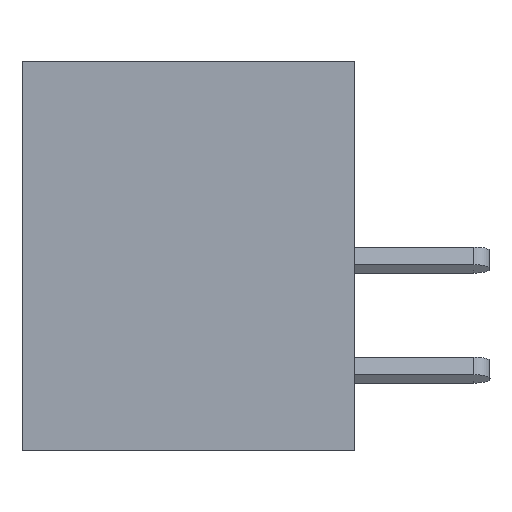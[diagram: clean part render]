
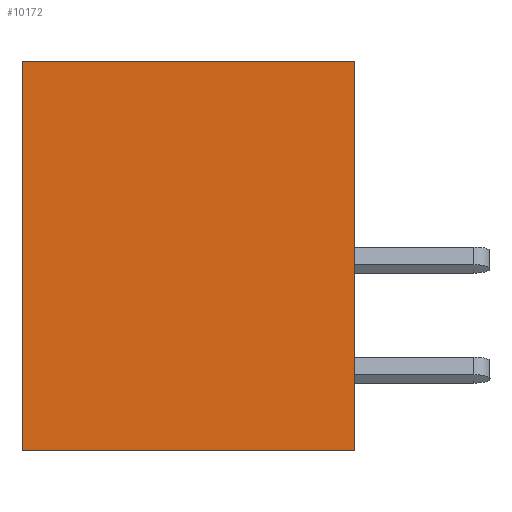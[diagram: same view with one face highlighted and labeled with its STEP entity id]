
A CAD part, left-side view. The second image highlights one B-rep face of the part: STEP entity #10172.
In plain terms, the highlighted planar face has unit normal (-1, 0, 0).
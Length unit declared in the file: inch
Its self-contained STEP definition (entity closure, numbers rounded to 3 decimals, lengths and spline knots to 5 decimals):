
#200 = CARTESIAN_POINT ( 'NONE',  ( 0., 0.453, 0. ) ) ;
#326 = LINE ( 'NONE', #12658, #6911 ) ;
#1226 = EDGE_CURVE ( 'NONE', #25572, #16957, #25368, .T. ) ;
#1540 = CARTESIAN_POINT ( 'NONE',  ( 0., 0.453, -0.531 ) ) ;
#1773 = CARTESIAN_POINT ( 'NONE',  ( 0., 0.453, 0. ) ) ;
#2562 = ORIENTED_EDGE ( 'NONE', *, *, #5221, .T. ) ;
#2761 = FACE_OUTER_BOUND ( 'NONE', #14135, .T. ) ;
#4261 = CARTESIAN_POINT ( 'NONE',  ( 0., 0.453, 0. ) ) ;
#5221 = EDGE_CURVE ( 'NONE', #15401, #17488, #27502, .T. ) ;
#6907 = DIRECTION ( 'NONE',  ( 0., -1., 0. ) ) ;
#6911 = VECTOR ( 'NONE', #14417, 39.37008 ) ;
#7282 = ORIENTED_EDGE ( 'NONE', *, *, #20754, .T. ) ;
#8296 = CARTESIAN_POINT ( 'NONE',  ( 0., 0., 0. ) ) ;
#10172 = ADVANCED_FACE ( 'NONE', ( #2761 ), #25554, .F. ) ;
#10483 = CARTESIAN_POINT ( 'NONE',  ( 0., 0.453, -0.531 ) ) ;
#11033 = ORIENTED_EDGE ( 'NONE', *, *, #1226, .F. ) ;
#12147 = VECTOR ( 'NONE', #6907, 39.37008 ) ;
#12658 = CARTESIAN_POINT ( 'NONE',  ( 0., 0., 0. ) ) ;
#12899 = DIRECTION ( 'NONE',  ( 0., 0., 1. ) ) ;
#14135 = EDGE_LOOP ( 'NONE', ( #7282, #11033, #19008, #2562 ) ) ;
#14417 = DIRECTION ( 'NONE',  ( 0., 0., 1. ) ) ;
#15272 = AXIS2_PLACEMENT_3D ( 'NONE', #20748, #21038, #18651 ) ;
#15401 = VERTEX_POINT ( 'NONE', #10483 ) ;
#15724 = VECTOR ( 'NONE', #18964, 39.37008 ) ;
#15932 = LINE ( 'NONE', #1773, #27024 ) ;
#16957 = VERTEX_POINT ( 'NONE', #8296 ) ;
#17488 = VERTEX_POINT ( 'NONE', #24282 ) ;
#18651 = DIRECTION ( 'NONE',  ( 0., 0., -1. ) ) ;
#18964 = DIRECTION ( 'NONE',  ( 0., -1., 0. ) ) ;
#19008 = ORIENTED_EDGE ( 'NONE', *, *, #26232, .F. ) ;
#20748 = CARTESIAN_POINT ( 'NONE',  ( 0., 0.453, 0. ) ) ;
#20754 = EDGE_CURVE ( 'NONE', #17488, #16957, #326, .T. ) ;
#21038 = DIRECTION ( 'NONE',  ( 1., 0., 0. ) ) ;
#24282 = CARTESIAN_POINT ( 'NONE',  ( 0., 0., -0.531 ) ) ;
#25368 = LINE ( 'NONE', #200, #12147 ) ;
#25554 = PLANE ( 'NONE',  #15272 ) ;
#25572 = VERTEX_POINT ( 'NONE', #4261 ) ;
#26232 = EDGE_CURVE ( 'NONE', #15401, #25572, #15932, .T. ) ;
#27024 = VECTOR ( 'NONE', #12899, 39.37008 ) ;
#27502 = LINE ( 'NONE', #1540, #15724 ) ;
